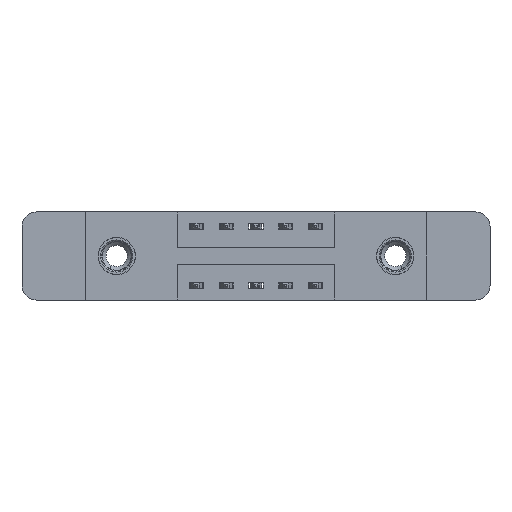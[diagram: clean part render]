
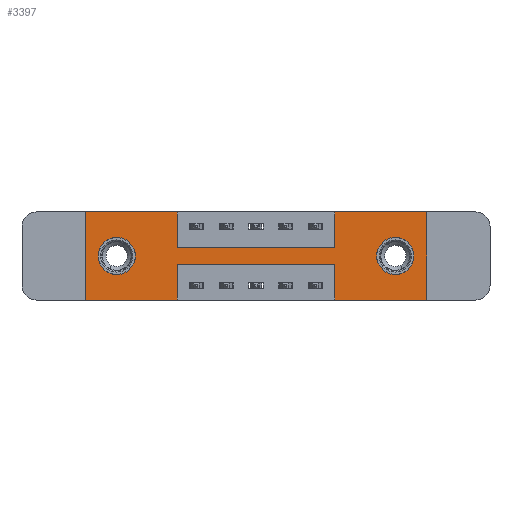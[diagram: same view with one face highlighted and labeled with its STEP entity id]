
A CAD part, front view. The second image highlights one B-rep face of the part: STEP entity #3397.
In plain terms, the highlighted planar face has unit normal (0, -1, 0).
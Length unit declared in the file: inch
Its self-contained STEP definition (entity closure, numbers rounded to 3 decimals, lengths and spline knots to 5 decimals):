
#233 = DIRECTION ( 'NONE',  ( 0., 1., 0. ) ) ;
#287 = FACE_BOUND ( 'NONE', #2583, .T. ) ;
#355 = LINE ( 'NONE', #10003, #8026 ) ;
#408 = CIRCLE ( 'NONE', #2118, 0.078 ) ;
#522 = PLANE ( 'NONE',  #6330 ) ;
#589 = VERTEX_POINT ( 'NONE', #3580 ) ;
#633 = CARTESIAN_POINT ( 'NONE',  ( 0.3875, 0., -0.37 ) ) ;
#667 = CARTESIAN_POINT ( 'NONE',  ( 0.3875, 0., 0. ) ) ;
#695 = VERTEX_POINT ( 'NONE', #2970 ) ;
#769 = DIRECTION ( 'NONE',  ( 0., 0., 1. ) ) ;
#973 = VECTOR ( 'NONE', #10490, 39.37008 ) ;
#1139 = ORIENTED_EDGE ( 'NONE', *, *, #12605, .T. ) ;
#1260 = CARTESIAN_POINT ( 'NONE',  ( 1.435, 0., -0.37 ) ) ;
#1310 = EDGE_CURVE ( 'NONE', #1730, #7607, #13262, .T. ) ;
#1467 = CARTESIAN_POINT ( 'NONE',  ( 0.3875, 0., -0.22 ) ) ;
#1498 = VECTOR ( 'NONE', #12767, 39.37008 ) ;
#1600 = ORIENTED_EDGE ( 'NONE', *, *, #1310, .F. ) ;
#1730 = VERTEX_POINT ( 'NONE', #10004 ) ;
#1767 = VERTEX_POINT ( 'NONE', #5871 ) ;
#1777 = VERTEX_POINT ( 'NONE', #5129 ) ;
#1875 = VECTOR ( 'NONE', #9845, 39.37008 ) ;
#1924 = CARTESIAN_POINT ( 'NONE',  ( 0.1325, 0., -0.185 ) ) ;
#1929 = EDGE_LOOP ( 'NONE', ( #9881, #4581, #12036, #11677, #9734, #6676, #8586, #7017, #7693, #1600, #6261, #5082 ) ) ;
#1959 = DIRECTION ( 'NONE',  ( 0., 1., 0. ) ) ;
#2022 = CARTESIAN_POINT ( 'NONE',  ( 1.435, 0., 0. ) ) ;
#2064 = EDGE_CURVE ( 'NONE', #8720, #1777, #12875, .T. ) ;
#2118 = AXIS2_PLACEMENT_3D ( 'NONE', #1924, #1959, #769 ) ;
#2139 = EDGE_CURVE ( 'NONE', #4167, #6988, #355, .T. ) ;
#2262 = DIRECTION ( 'NONE',  ( 0., 0., -1. ) ) ;
#2380 = CIRCLE ( 'NONE', #4111, 0.078 ) ;
#2423 = VERTEX_POINT ( 'NONE', #12689 ) ;
#2504 = CARTESIAN_POINT ( 'NONE',  ( 0.3875, 0., -0.37 ) ) ;
#2583 = EDGE_LOOP ( 'NONE', ( #8886, #5626 ) ) ;
#2619 = CIRCLE ( 'NONE', #5100, 0.078 ) ;
#2869 = DIRECTION ( 'NONE',  ( -1., 0., 0. ) ) ;
#2933 = VECTOR ( 'NONE', #12142, 39.37008 ) ;
#2970 = CARTESIAN_POINT ( 'NONE',  ( 1.0475, 0., 0. ) ) ;
#3053 = CARTESIAN_POINT ( 'NONE',  ( 0., 0., 0. ) ) ;
#3187 = VERTEX_POINT ( 'NONE', #4793 ) ;
#3272 = VECTOR ( 'NONE', #9334, 39.37008 ) ;
#3397 = ADVANCED_FACE ( 'NONE', ( #9249, #287, #8137 ), #522, .T. ) ;
#3580 = CARTESIAN_POINT ( 'NONE',  ( 0.3875, 0., -0.22 ) ) ;
#3704 = DIRECTION ( 'NONE',  ( 0., 1., 0. ) ) ;
#3833 = DIRECTION ( 'NONE',  ( -1., 0., 0. ) ) ;
#3954 = VECTOR ( 'NONE', #5916, 39.37008 ) ;
#4084 = EDGE_CURVE ( 'NONE', #589, #8720, #5174, .T. ) ;
#4097 = EDGE_LOOP ( 'NONE', ( #1139, #9212 ) ) ;
#4111 = AXIS2_PLACEMENT_3D ( 'NONE', #10415, #10471, #5141 ) ;
#4167 = VERTEX_POINT ( 'NONE', #1260 ) ;
#4569 = LINE ( 'NONE', #3053, #3954 ) ;
#4581 = ORIENTED_EDGE ( 'NONE', *, *, #13334, .F. ) ;
#4667 = DIRECTION ( 'NONE',  ( 0., 0., -1. ) ) ;
#4793 = CARTESIAN_POINT ( 'NONE',  ( 1.3025, 0., -0.107 ) ) ;
#4861 = CARTESIAN_POINT ( 'NONE',  ( 0., 0., 0. ) ) ;
#4959 = DIRECTION ( 'NONE',  ( 0., 0., -1. ) ) ;
#5082 = ORIENTED_EDGE ( 'NONE', *, *, #2064, .F. ) ;
#5100 = AXIS2_PLACEMENT_3D ( 'NONE', #11838, #233, #9606 ) ;
#5129 = CARTESIAN_POINT ( 'NONE',  ( 0., 0., -0.37 ) ) ;
#5141 = DIRECTION ( 'NONE',  ( 0., 0., -1. ) ) ;
#5174 = LINE ( 'NONE', #2504, #6301 ) ;
#5581 = VERTEX_POINT ( 'NONE', #8161 ) ;
#5626 = ORIENTED_EDGE ( 'NONE', *, *, #10400, .T. ) ;
#5871 = CARTESIAN_POINT ( 'NONE',  ( 1.0475, 0., -0.22 ) ) ;
#5916 = DIRECTION ( 'NONE',  ( 0., 0., 1. ) ) ;
#6261 = ORIENTED_EDGE ( 'NONE', *, *, #11210, .F. ) ;
#6301 = VECTOR ( 'NONE', #12845, 39.37008 ) ;
#6330 = AXIS2_PLACEMENT_3D ( 'NONE', #9993, #7812, #4667 ) ;
#6590 = EDGE_CURVE ( 'NONE', #5581, #3187, #2380, .T. ) ;
#6676 = ORIENTED_EDGE ( 'NONE', *, *, #6941, .F. ) ;
#6698 = EDGE_CURVE ( 'NONE', #7607, #7583, #7561, .T. ) ;
#6726 = CARTESIAN_POINT ( 'NONE',  ( 0., 0., -0.37 ) ) ;
#6741 = CARTESIAN_POINT ( 'NONE',  ( 0.3875, 0., -0.15 ) ) ;
#6760 = LINE ( 'NONE', #2022, #11941 ) ;
#6765 = CIRCLE ( 'NONE', #12985, 0.078 ) ;
#6828 = EDGE_CURVE ( 'NONE', #10843, #4167, #6760, .T. ) ;
#6941 = EDGE_CURVE ( 'NONE', #695, #10843, #7498, .T. ) ;
#6988 = VERTEX_POINT ( 'NONE', #10251 ) ;
#7017 = ORIENTED_EDGE ( 'NONE', *, *, #10586, .F. ) ;
#7498 = LINE ( 'NONE', #4861, #9442 ) ;
#7551 = VECTOR ( 'NONE', #2869, 39.37008 ) ;
#7561 = LINE ( 'NONE', #9453, #8680 ) ;
#7583 = VERTEX_POINT ( 'NONE', #6741 ) ;
#7607 = VERTEX_POINT ( 'NONE', #667 ) ;
#7693 = ORIENTED_EDGE ( 'NONE', *, *, #6698, .F. ) ;
#7812 = DIRECTION ( 'NONE',  ( 0., -1., 0. ) ) ;
#7839 = EDGE_CURVE ( 'NONE', #6988, #1767, #9577, .T. ) ;
#7946 = VERTEX_POINT ( 'NONE', #11058 ) ;
#8026 = VECTOR ( 'NONE', #3833, 39.37008 ) ;
#8137 = FACE_OUTER_BOUND ( 'NONE', #1929, .T. ) ;
#8161 = CARTESIAN_POINT ( 'NONE',  ( 1.3025, 0., -0.263 ) ) ;
#8469 = LINE ( 'NONE', #11745, #1498 ) ;
#8586 = ORIENTED_EDGE ( 'NONE', *, *, #10098, .F. ) ;
#8680 = VECTOR ( 'NONE', #2262, 39.37008 ) ;
#8720 = VERTEX_POINT ( 'NONE', #633 ) ;
#8886 = ORIENTED_EDGE ( 'NONE', *, *, #8962, .T. ) ;
#8962 = EDGE_CURVE ( 'NONE', #2423, #10470, #408, .T. ) ;
#9086 = CARTESIAN_POINT ( 'NONE',  ( 0.3875, 0., -0.15 ) ) ;
#9212 = ORIENTED_EDGE ( 'NONE', *, *, #6590, .T. ) ;
#9249 = FACE_BOUND ( 'NONE', #4097, .T. ) ;
#9334 = DIRECTION ( 'NONE',  ( 1., 0., 0. ) ) ;
#9442 = VECTOR ( 'NONE', #13149, 39.37008 ) ;
#9453 = CARTESIAN_POINT ( 'NONE',  ( 0.3875, 0., 0. ) ) ;
#9577 = LINE ( 'NONE', #10663, #973 ) ;
#9606 = DIRECTION ( 'NONE',  ( 0., 0., 1. ) ) ;
#9734 = ORIENTED_EDGE ( 'NONE', *, *, #6828, .F. ) ;
#9845 = DIRECTION ( 'NONE',  ( -1., 0., 0. ) ) ;
#9881 = ORIENTED_EDGE ( 'NONE', *, *, #4084, .F. ) ;
#9993 = CARTESIAN_POINT ( 'NONE',  ( 0., 0., -0.37 ) ) ;
#10003 = CARTESIAN_POINT ( 'NONE',  ( 0., 0., -0.37 ) ) ;
#10004 = CARTESIAN_POINT ( 'NONE',  ( 0., 0., 0. ) ) ;
#10098 = EDGE_CURVE ( 'NONE', #7946, #695, #8469, .T. ) ;
#10251 = CARTESIAN_POINT ( 'NONE',  ( 1.0475, 0., -0.37 ) ) ;
#10400 = EDGE_CURVE ( 'NONE', #10470, #2423, #2619, .T. ) ;
#10415 = CARTESIAN_POINT ( 'NONE',  ( 1.3025, 0., -0.185 ) ) ;
#10470 = VERTEX_POINT ( 'NONE', #13030 ) ;
#10471 = DIRECTION ( 'NONE',  ( 0., 1., 0. ) ) ;
#10490 = DIRECTION ( 'NONE',  ( 0., 0., 1. ) ) ;
#10557 = CARTESIAN_POINT ( 'NONE',  ( 1.435, 0., 0. ) ) ;
#10586 = EDGE_CURVE ( 'NONE', #7583, #7946, #12297, .T. ) ;
#10663 = CARTESIAN_POINT ( 'NONE',  ( 1.0475, 0., -0.37 ) ) ;
#10843 = VERTEX_POINT ( 'NONE', #10557 ) ;
#10890 = CARTESIAN_POINT ( 'NONE',  ( 1.3025, 0., -0.185 ) ) ;
#11058 = CARTESIAN_POINT ( 'NONE',  ( 1.0475, 0., -0.15 ) ) ;
#11210 = EDGE_CURVE ( 'NONE', #1777, #1730, #4569, .T. ) ;
#11677 = ORIENTED_EDGE ( 'NONE', *, *, #2139, .F. ) ;
#11745 = CARTESIAN_POINT ( 'NONE',  ( 1.0475, 0., 0. ) ) ;
#11838 = CARTESIAN_POINT ( 'NONE',  ( 0.1325, 0., -0.185 ) ) ;
#11941 = VECTOR ( 'NONE', #4959, 39.37008 ) ;
#12001 = DIRECTION ( 'NONE',  ( 0., 0., -1. ) ) ;
#12036 = ORIENTED_EDGE ( 'NONE', *, *, #7839, .F. ) ;
#12142 = DIRECTION ( 'NONE',  ( 1., 0., 0. ) ) ;
#12297 = LINE ( 'NONE', #9086, #2933 ) ;
#12605 = EDGE_CURVE ( 'NONE', #3187, #5581, #6765, .T. ) ;
#12689 = CARTESIAN_POINT ( 'NONE',  ( 0.1325, 0., -0.107 ) ) ;
#12767 = DIRECTION ( 'NONE',  ( 0., 0., 1. ) ) ;
#12845 = DIRECTION ( 'NONE',  ( 0., 0., -1. ) ) ;
#12875 = LINE ( 'NONE', #6726, #1875 ) ;
#12985 = AXIS2_PLACEMENT_3D ( 'NONE', #10890, #3704, #12001 ) ;
#13030 = CARTESIAN_POINT ( 'NONE',  ( 0.1325, 0., -0.263 ) ) ;
#13062 = LINE ( 'NONE', #1467, #7551 ) ;
#13149 = DIRECTION ( 'NONE',  ( 1., 0., 0. ) ) ;
#13262 = LINE ( 'NONE', #13414, #3272 ) ;
#13334 = EDGE_CURVE ( 'NONE', #1767, #589, #13062, .T. ) ;
#13414 = CARTESIAN_POINT ( 'NONE',  ( 0., 0., 0. ) ) ;
